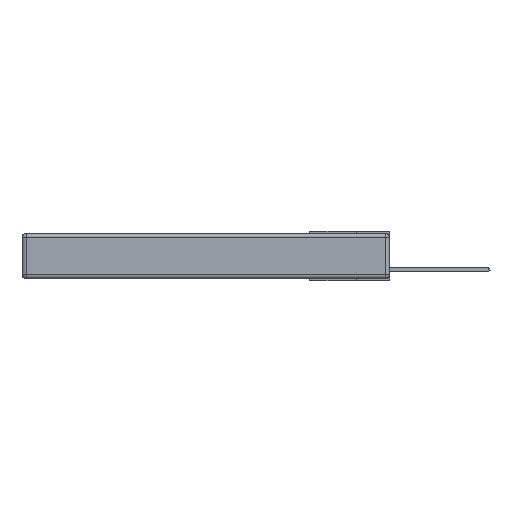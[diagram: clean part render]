
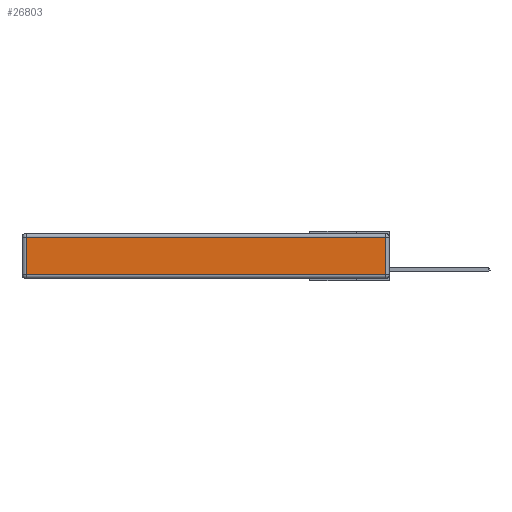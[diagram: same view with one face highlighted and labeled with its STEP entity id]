
A CAD part, left-side view. The second image highlights one B-rep face of the part: STEP entity #26803.
In plain terms, the highlighted planar face has unit normal (-1, 0, 0).
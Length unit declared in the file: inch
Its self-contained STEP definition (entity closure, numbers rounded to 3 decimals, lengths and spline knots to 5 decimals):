
#287 = VERTEX_POINT ( 'NONE', #28832 ) ;
#291 = VECTOR ( 'NONE', #26830, 39.37008 ) ;
#786 = AXIS2_PLACEMENT_3D ( 'NONE', #17320, #17423, #24770 ) ;
#1496 = CARTESIAN_POINT ( 'NONE',  ( 0., 2.72, -0.313 ) ) ;
#2134 = LINE ( 'NONE', #15790, #9220 ) ;
#2176 = LINE ( 'NONE', #6311, #17129 ) ;
#2578 = ORIENTED_EDGE ( 'NONE', *, *, #4187, .T. ) ;
#4187 = EDGE_CURVE ( 'NONE', #18955, #13417, #16878, .T. ) ;
#6311 = CARTESIAN_POINT ( 'NONE',  ( 0., 0.03, -0.343 ) ) ;
#6483 = EDGE_CURVE ( 'NONE', #13417, #287, #2176, .T. ) ;
#6641 = CARTESIAN_POINT ( 'NONE',  ( 0., 2.72, -0.343 ) ) ;
#6693 = DIRECTION ( 'NONE',  ( 0., -1., 0. ) ) ;
#7115 = ORIENTED_EDGE ( 'NONE', *, *, #6483, .T. ) ;
#7888 = CARTESIAN_POINT ( 'NONE',  ( 0., 0.03, -0.313 ) ) ;
#8629 = VECTOR ( 'NONE', #6693, 39.37008 ) ;
#8801 = ORIENTED_EDGE ( 'NONE', *, *, #25448, .T. ) ;
#9220 = VECTOR ( 'NONE', #25740, 39.37008 ) ;
#11177 = EDGE_CURVE ( 'NONE', #25498, #18955, #27032, .T. ) ;
#13417 = VERTEX_POINT ( 'NONE', #7888 ) ;
#15790 = CARTESIAN_POINT ( 'NONE',  ( 0., 2.75, -0.03 ) ) ;
#16331 = DIRECTION ( 'NONE',  ( 0., 0., 1. ) ) ;
#16878 = LINE ( 'NONE', #21485, #8629 ) ;
#17129 = VECTOR ( 'NONE', #16331, 39.37008 ) ;
#17320 = CARTESIAN_POINT ( 'NONE',  ( 0., 0., -0.343 ) ) ;
#17423 = DIRECTION ( 'NONE',  ( -1., 0., 0. ) ) ;
#17511 = EDGE_LOOP ( 'NONE', ( #2578, #7115, #8801, #29009 ) ) ;
#17948 = CARTESIAN_POINT ( 'NONE',  ( 0., 2.72, -0.03 ) ) ;
#18955 = VERTEX_POINT ( 'NONE', #1496 ) ;
#21485 = CARTESIAN_POINT ( 'NONE',  ( 0., 0., -0.313 ) ) ;
#24770 = DIRECTION ( 'NONE',  ( 0., 0., 1. ) ) ;
#25101 = PLANE ( 'NONE',  #786 ) ;
#25448 = EDGE_CURVE ( 'NONE', #287, #25498, #2134, .T. ) ;
#25498 = VERTEX_POINT ( 'NONE', #17948 ) ;
#25740 = DIRECTION ( 'NONE',  ( 0., 1., 0. ) ) ;
#26803 = ADVANCED_FACE ( 'NONE', ( #27165 ), #25101, .T. ) ;
#26830 = DIRECTION ( 'NONE',  ( 0., 0., -1. ) ) ;
#27032 = LINE ( 'NONE', #6641, #291 ) ;
#27165 = FACE_OUTER_BOUND ( 'NONE', #17511, .T. ) ;
#28832 = CARTESIAN_POINT ( 'NONE',  ( 0., 0.03, -0.03 ) ) ;
#29009 = ORIENTED_EDGE ( 'NONE', *, *, #11177, .T. ) ;
